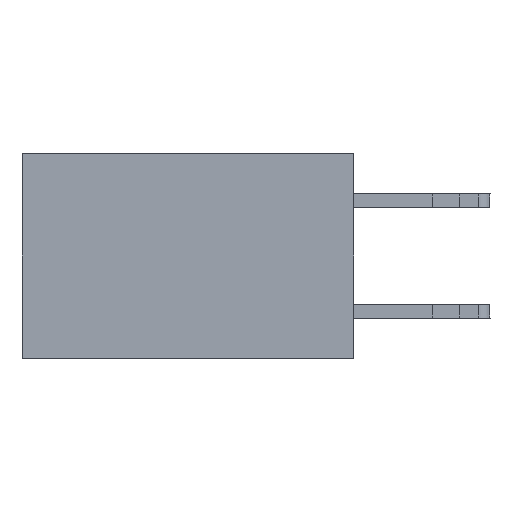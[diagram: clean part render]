
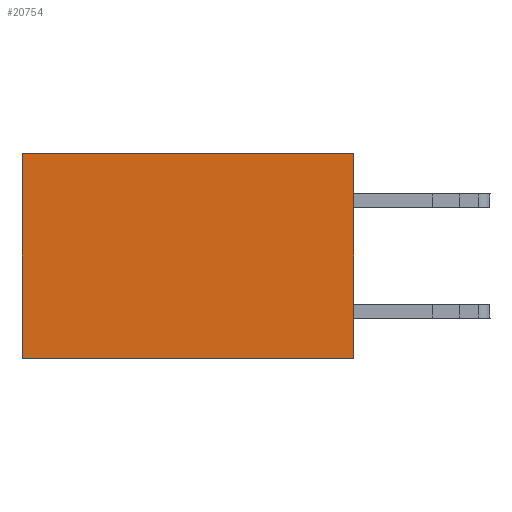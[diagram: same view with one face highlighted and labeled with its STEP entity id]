
A CAD part, left-side view. The second image highlights one B-rep face of the part: STEP entity #20754.
In plain terms, the highlighted planar face has unit normal (-1, 0, 0).
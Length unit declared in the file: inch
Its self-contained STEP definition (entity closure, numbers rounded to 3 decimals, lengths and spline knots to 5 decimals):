
#1129 = ORIENTED_EDGE ( 'NONE', *, *, #4712, .F. ) ;
#2202 = DIRECTION ( 'NONE',  ( 0., 1., 0. ) ) ;
#2560 = VECTOR ( 'NONE', #10069, 39.37008 ) ;
#2904 = VERTEX_POINT ( 'NONE', #30974 ) ;
#3541 = EDGE_CURVE ( 'NONE', #24987, #15546, #34230, .T. ) ;
#4712 = EDGE_CURVE ( 'NONE', #2904, #24987, #21887, .T. ) ;
#6812 = EDGE_CURVE ( 'NONE', #21420, #15546, #24688, .T. ) ;
#7703 = VECTOR ( 'NONE', #33755, 39.37008 ) ;
#8594 = FACE_OUTER_BOUND ( 'NONE', #20830, .T. ) ;
#10069 = DIRECTION ( 'NONE',  ( 0., 1., 0. ) ) ;
#10170 = CARTESIAN_POINT ( 'NONE',  ( 0.2875, 0.6, 0. ) ) ;
#11658 = CARTESIAN_POINT ( 'NONE',  ( 0.2875, 0., -0.37 ) ) ;
#13492 = ORIENTED_EDGE ( 'NONE', *, *, #6812, .T. ) ;
#13611 = DIRECTION ( 'NONE',  ( 0., 0., -1. ) ) ;
#15546 = VERTEX_POINT ( 'NONE', #20670 ) ;
#15806 = DIRECTION ( 'NONE',  ( 1., 0., 0. ) ) ;
#16654 = VECTOR ( 'NONE', #2202, 39.37008 ) ;
#20490 = LINE ( 'NONE', #28751, #2560 ) ;
#20670 = CARTESIAN_POINT ( 'NONE',  ( 0.2875, 0.6, -0.37 ) ) ;
#20754 = ADVANCED_FACE ( 'NONE', ( #8594 ), #21496, .F. ) ;
#20830 = EDGE_LOOP ( 'NONE', ( #13492, #27063, #1129, #32886 ) ) ;
#20919 = VECTOR ( 'NONE', #32936, 39.37008 ) ;
#21420 = VERTEX_POINT ( 'NONE', #10170 ) ;
#21496 = PLANE ( 'NONE',  #32162 ) ;
#21887 = LINE ( 'NONE', #33339, #7703 ) ;
#23763 = CARTESIAN_POINT ( 'NONE',  ( 0.2875, 0., -0.37 ) ) ;
#23956 = CARTESIAN_POINT ( 'NONE',  ( 0.2875, 0., 0. ) ) ;
#23965 = EDGE_CURVE ( 'NONE', #2904, #21420, #20490, .T. ) ;
#24688 = LINE ( 'NONE', #30148, #20919 ) ;
#24987 = VERTEX_POINT ( 'NONE', #11658 ) ;
#27063 = ORIENTED_EDGE ( 'NONE', *, *, #3541, .F. ) ;
#28751 = CARTESIAN_POINT ( 'NONE',  ( 0.2875, 0., 0. ) ) ;
#30148 = CARTESIAN_POINT ( 'NONE',  ( 0.2875, 0.6, 0. ) ) ;
#30974 = CARTESIAN_POINT ( 'NONE',  ( 0.2875, 0., 0. ) ) ;
#32162 = AXIS2_PLACEMENT_3D ( 'NONE', #23956, #15806, #13611 ) ;
#32886 = ORIENTED_EDGE ( 'NONE', *, *, #23965, .T. ) ;
#32936 = DIRECTION ( 'NONE',  ( 0., 0., -1. ) ) ;
#33339 = CARTESIAN_POINT ( 'NONE',  ( 0.2875, 0., 0. ) ) ;
#33755 = DIRECTION ( 'NONE',  ( 0., 0., -1. ) ) ;
#34230 = LINE ( 'NONE', #23763, #16654 ) ;
